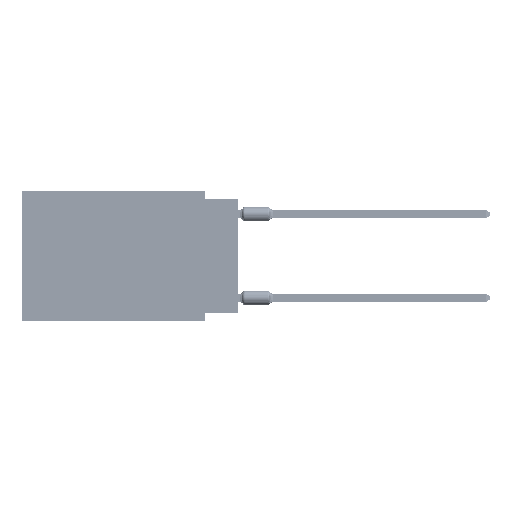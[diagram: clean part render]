
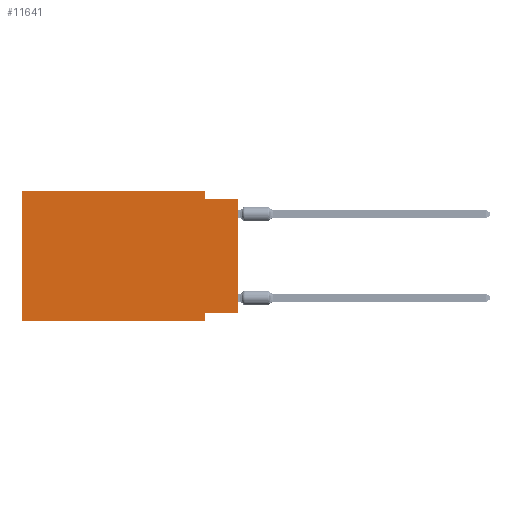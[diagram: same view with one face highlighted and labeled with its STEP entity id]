
A CAD part, left-side view. The second image highlights one B-rep face of the part: STEP entity #11641.
In plain terms, the highlighted planar face has unit normal (-1, 0, 0).
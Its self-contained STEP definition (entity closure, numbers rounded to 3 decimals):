
#1029 = CARTESIAN_POINT ( 'NONE',  ( 0., 2.54, 0. ) ) ;
#1286 = VERTEX_POINT ( 'NONE', #43001 ) ;
#1867 = CARTESIAN_POINT ( 'NONE',  ( 0., 0., 0. ) ) ;
#1902 = CARTESIAN_POINT ( 'NONE',  ( 0., 2.54, -9.271 ) ) ;
#4286 = AXIS2_PLACEMENT_3D ( 'NONE', #7732, #34280, #65363 ) ;
#4292 = VERTEX_POINT ( 'NONE', #42545 ) ;
#7732 = CARTESIAN_POINT ( 'NONE',  ( 0., 16.383, 0. ) ) ;
#7897 = DIRECTION ( 'NONE',  ( 0., 0., -1. ) ) ;
#8395 = CARTESIAN_POINT ( 'NONE',  ( 0., 16.383, 0. ) ) ;
#10391 = ORIENTED_EDGE ( 'NONE', *, *, #12027, .F. ) ;
#11308 = VECTOR ( 'NONE', #30588, 1000. ) ;
#11604 = FACE_OUTER_BOUND ( 'NONE', #23175, .T. ) ;
#11641 = ADVANCED_FACE ( 'NONE', ( #11604 ), #44411, .F. ) ;
#12027 = EDGE_CURVE ( 'NONE', #48718, #43812, #54370, .T. ) ;
#15360 = DIRECTION ( 'NONE',  ( 0., -1., 0. ) ) ;
#15774 = VERTEX_POINT ( 'NONE', #16978 ) ;
#16247 = VECTOR ( 'NONE', #49346, 1000. ) ;
#16882 = CARTESIAN_POINT ( 'NONE',  ( 0., 0., -9.271 ) ) ;
#16978 = CARTESIAN_POINT ( 'NONE',  ( 0., 2.54, -0.635 ) ) ;
#18730 = LINE ( 'NONE', #29197, #54072 ) ;
#18838 = EDGE_CURVE ( 'NONE', #48718, #1286, #38874, .T. ) ;
#19200 = DIRECTION ( 'NONE',  ( 0., -1., 0. ) ) ;
#19627 = EDGE_CURVE ( 'NONE', #4292, #45438, #44633, .T. ) ;
#22306 = CARTESIAN_POINT ( 'NONE',  ( 0., 16.383, -9.906 ) ) ;
#22598 = DIRECTION ( 'NONE',  ( 0., 1., 0. ) ) ;
#23175 = EDGE_LOOP ( 'NONE', ( #50929, #50953, #45179, #45673, #49630, #63803, #53262, #10391 ) ) ;
#26523 = CARTESIAN_POINT ( 'NONE',  ( 0., 0., -0.635 ) ) ;
#29197 = CARTESIAN_POINT ( 'NONE',  ( 0., 2.54, 0. ) ) ;
#30354 = VECTOR ( 'NONE', #19200, 1000. ) ;
#30588 = DIRECTION ( 'NONE',  ( 0., 0., -1. ) ) ;
#30740 = CARTESIAN_POINT ( 'NONE',  ( 0., 16.383, 0. ) ) ;
#30933 = CARTESIAN_POINT ( 'NONE',  ( 0., 2.54, -9.906 ) ) ;
#33065 = VECTOR ( 'NONE', #51007, 1000. ) ;
#34280 = DIRECTION ( 'NONE',  ( 1., 0., 0. ) ) ;
#38714 = DIRECTION ( 'NONE',  ( 0., -1., 0. ) ) ;
#38874 = LINE ( 'NONE', #1867, #16247 ) ;
#38996 = CARTESIAN_POINT ( 'NONE',  ( 0., 16.383, 0. ) ) ;
#42545 = CARTESIAN_POINT ( 'NONE',  ( 0., 16.383, -9.906 ) ) ;
#43001 = CARTESIAN_POINT ( 'NONE',  ( 0., 0., -0.635 ) ) ;
#43540 = CARTESIAN_POINT ( 'NONE',  ( 0., 0., -9.271 ) ) ;
#43812 = VERTEX_POINT ( 'NONE', #1902 ) ;
#44411 = PLANE ( 'NONE',  #4286 ) ;
#44633 = LINE ( 'NONE', #22306, #50887 ) ;
#45179 = ORIENTED_EDGE ( 'NONE', *, *, #55243, .F. ) ;
#45438 = VERTEX_POINT ( 'NONE', #66748 ) ;
#45673 = ORIENTED_EDGE ( 'NONE', *, *, #52245, .F. ) ;
#46094 = LINE ( 'NONE', #8395, #30354 ) ;
#46947 = VECTOR ( 'NONE', #15360, 1000. ) ;
#48718 = VERTEX_POINT ( 'NONE', #16882 ) ;
#49346 = DIRECTION ( 'NONE',  ( 0., 0., 1. ) ) ;
#49630 = ORIENTED_EDGE ( 'NONE', *, *, #58401, .F. ) ;
#50887 = VECTOR ( 'NONE', #38714, 1000. ) ;
#50929 = ORIENTED_EDGE ( 'NONE', *, *, #18838, .T. ) ;
#50953 = ORIENTED_EDGE ( 'NONE', *, *, #66996, .F. ) ;
#51007 = DIRECTION ( 'NONE',  ( 0., 0., 1. ) ) ;
#51537 = EDGE_CURVE ( 'NONE', #43812, #45438, #57805, .T. ) ;
#52236 = VECTOR ( 'NONE', #22598, 1000. ) ;
#52245 = EDGE_CURVE ( 'NONE', #55365, #54778, #46094, .T. ) ;
#52709 = LINE ( 'NONE', #26523, #46947 ) ;
#53262 = ORIENTED_EDGE ( 'NONE', *, *, #51537, .F. ) ;
#54072 = VECTOR ( 'NONE', #7897, 1000. ) ;
#54370 = LINE ( 'NONE', #43540, #52236 ) ;
#54778 = VERTEX_POINT ( 'NONE', #1029 ) ;
#55243 = EDGE_CURVE ( 'NONE', #54778, #15774, #18730, .T. ) ;
#55365 = VERTEX_POINT ( 'NONE', #38996 ) ;
#57805 = LINE ( 'NONE', #30933, #11308 ) ;
#58401 = EDGE_CURVE ( 'NONE', #4292, #55365, #67410, .T. ) ;
#63803 = ORIENTED_EDGE ( 'NONE', *, *, #19627, .T. ) ;
#65363 = DIRECTION ( 'NONE',  ( 0., 0., -1. ) ) ;
#66748 = CARTESIAN_POINT ( 'NONE',  ( 0., 2.54, -9.906 ) ) ;
#66996 = EDGE_CURVE ( 'NONE', #15774, #1286, #52709, .T. ) ;
#67410 = LINE ( 'NONE', #30740, #33065 ) ;
